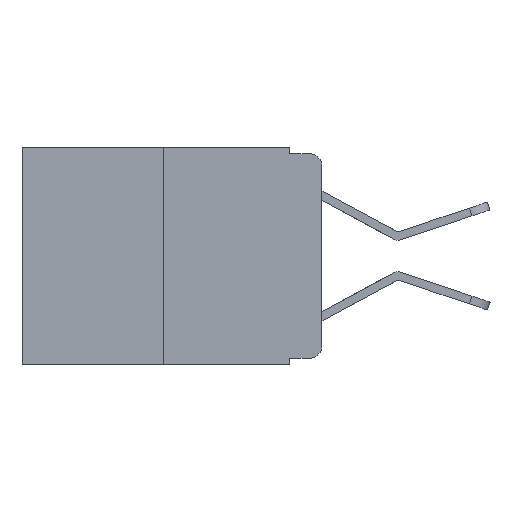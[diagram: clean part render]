
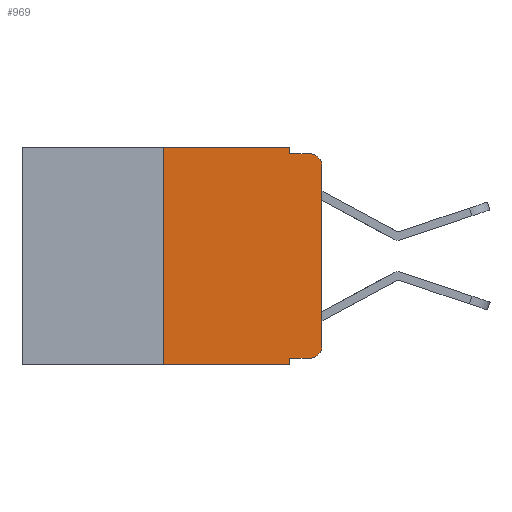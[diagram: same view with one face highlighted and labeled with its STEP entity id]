
A CAD part, left-side view. The second image highlights one B-rep face of the part: STEP entity #969.
In plain terms, the highlighted planar face has unit normal (-1, 0, 0).
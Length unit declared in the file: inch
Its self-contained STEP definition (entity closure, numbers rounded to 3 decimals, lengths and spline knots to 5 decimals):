
#143 = VECTOR ( 'NONE', #13954, 39.37008 ) ;
#254 = LINE ( 'NONE', #5528, #7622 ) ;
#380 = CARTESIAN_POINT ( 'NONE',  ( 0., 0.25, 0. ) ) ;
#518 = LINE ( 'NONE', #10164, #143 ) ;
#664 = VERTEX_POINT ( 'NONE', #6516 ) ;
#759 = AXIS2_PLACEMENT_3D ( 'NONE', #9137, #15104, #14919 ) ;
#808 = LINE ( 'NONE', #10025, #13020 ) ;
#903 = PLANE ( 'NONE',  #759 ) ;
#969 = ADVANCED_FACE ( 'NONE', ( #3757 ), #903, .F. ) ;
#1023 = CARTESIAN_POINT ( 'NONE',  ( 0., 0.051, 0. ) ) ;
#1136 = EDGE_CURVE ( 'NONE', #5374, #13135, #7244, .T. ) ;
#1180 = ORIENTED_EDGE ( 'NONE', *, *, #13018, .T. ) ;
#1422 = LINE ( 'NONE', #1023, #13125 ) ;
#3008 = CARTESIAN_POINT ( 'NONE',  ( 0., 0.02, -0.333 ) ) ;
#3103 = CIRCLE ( 'NONE', #9961, 0.02 ) ;
#3484 = CARTESIAN_POINT ( 'NONE',  ( 0., 0.051, -0.333 ) ) ;
#3704 = EDGE_CURVE ( 'NONE', #8848, #664, #3103, .T. ) ;
#3757 = FACE_OUTER_BOUND ( 'NONE', #5699, .T. ) ;
#3791 = VECTOR ( 'NONE', #14835, 39.37008 ) ;
#3911 = CARTESIAN_POINT ( 'NONE',  ( 0., 0.051, -0.01 ) ) ;
#3981 = EDGE_CURVE ( 'NONE', #11200, #5374, #14422, .T. ) ;
#4376 = DIRECTION ( 'NONE',  ( 0., 0., 1. ) ) ;
#4442 = EDGE_CURVE ( 'NONE', #4542, #13121, #1422, .T. ) ;
#4503 = LINE ( 'NONE', #380, #15077 ) ;
#4542 = VERTEX_POINT ( 'NONE', #3484 ) ;
#5076 = VECTOR ( 'NONE', #13237, 39.37008 ) ;
#5219 = VERTEX_POINT ( 'NONE', #9619 ) ;
#5374 = VERTEX_POINT ( 'NONE', #3911 ) ;
#5528 = CARTESIAN_POINT ( 'NONE',  ( 0., 0., 0. ) ) ;
#5699 = EDGE_LOOP ( 'NONE', ( #10292, #7674, #13371, #15097, #11993, #7502, #1180, #9993, #12969, #14958 ) ) ;
#6398 = CIRCLE ( 'NONE', #10613, 0.02 ) ;
#6484 = EDGE_CURVE ( 'NONE', #7038, #7924, #4503, .T. ) ;
#6516 = CARTESIAN_POINT ( 'NONE',  ( 0., 0., -0.313 ) ) ;
#6709 = LINE ( 'NONE', #12533, #3791 ) ;
#7038 = VERTEX_POINT ( 'NONE', #8792 ) ;
#7244 = LINE ( 'NONE', #12043, #5076 ) ;
#7458 = CARTESIAN_POINT ( 'NONE',  ( 0., 0.25, 0. ) ) ;
#7502 = ORIENTED_EDGE ( 'NONE', *, *, #6484, .F. ) ;
#7622 = VECTOR ( 'NONE', #4376, 39.37008 ) ;
#7674 = ORIENTED_EDGE ( 'NONE', *, *, #11751, .T. ) ;
#7924 = VERTEX_POINT ( 'NONE', #7458 ) ;
#8792 = CARTESIAN_POINT ( 'NONE',  ( 0., 0.25, -0.343 ) ) ;
#8848 = VERTEX_POINT ( 'NONE', #3008 ) ;
#8976 = DIRECTION ( 'NONE',  ( -1., 0., 0. ) ) ;
#9137 = CARTESIAN_POINT ( 'NONE',  ( 0., 0.473, 0. ) ) ;
#9619 = CARTESIAN_POINT ( 'NONE',  ( 0., 0., -0.03 ) ) ;
#9640 = DIRECTION ( 'NONE',  ( -1., 0., 0. ) ) ;
#9930 = CARTESIAN_POINT ( 'NONE',  ( 0., 0.051, 0. ) ) ;
#9961 = AXIS2_PLACEMENT_3D ( 'NONE', #10929, #9640, #10818 ) ;
#9993 = ORIENTED_EDGE ( 'NONE', *, *, #4442, .F. ) ;
#10025 = CARTESIAN_POINT ( 'NONE',  ( 0., 0.051, -0.333 ) ) ;
#10082 = EDGE_CURVE ( 'NONE', #7924, #11200, #518, .T. ) ;
#10164 = CARTESIAN_POINT ( 'NONE',  ( 0., 0.473, 0. ) ) ;
#10254 = CARTESIAN_POINT ( 'NONE',  ( 0., 0.02, -0.03 ) ) ;
#10292 = ORIENTED_EDGE ( 'NONE', *, *, #13781, .T. ) ;
#10613 = AXIS2_PLACEMENT_3D ( 'NONE', #10254, #8976, #15006 ) ;
#10818 = DIRECTION ( 'NONE',  ( 0., 0., -1. ) ) ;
#10929 = CARTESIAN_POINT ( 'NONE',  ( 0., 0.02, -0.313 ) ) ;
#11200 = VERTEX_POINT ( 'NONE', #14034 ) ;
#11751 = EDGE_CURVE ( 'NONE', #5219, #13135, #6398, .T. ) ;
#11993 = ORIENTED_EDGE ( 'NONE', *, *, #10082, .F. ) ;
#12043 = CARTESIAN_POINT ( 'NONE',  ( 0., 0.051, -0.01 ) ) ;
#12533 = CARTESIAN_POINT ( 'NONE',  ( 0., 0.473, -0.343 ) ) ;
#12588 = CARTESIAN_POINT ( 'NONE',  ( 0., 0.02, -0.01 ) ) ;
#12664 = DIRECTION ( 'NONE',  ( 0., 0., -1. ) ) ;
#12969 = ORIENTED_EDGE ( 'NONE', *, *, #13627, .T. ) ;
#13018 = EDGE_CURVE ( 'NONE', #7038, #13121, #6709, .T. ) ;
#13020 = VECTOR ( 'NONE', #13435, 39.37008 ) ;
#13121 = VERTEX_POINT ( 'NONE', #13988 ) ;
#13125 = VECTOR ( 'NONE', #12664, 39.37008 ) ;
#13135 = VERTEX_POINT ( 'NONE', #12588 ) ;
#13200 = DIRECTION ( 'NONE',  ( 0., 0., 1. ) ) ;
#13237 = DIRECTION ( 'NONE',  ( 0., -1., 0. ) ) ;
#13371 = ORIENTED_EDGE ( 'NONE', *, *, #1136, .F. ) ;
#13435 = DIRECTION ( 'NONE',  ( 0., -1., 0. ) ) ;
#13627 = EDGE_CURVE ( 'NONE', #4542, #8848, #808, .T. ) ;
#13781 = EDGE_CURVE ( 'NONE', #664, #5219, #254, .T. ) ;
#13848 = VECTOR ( 'NONE', #14646, 39.37008 ) ;
#13954 = DIRECTION ( 'NONE',  ( 0., -1., 0. ) ) ;
#13988 = CARTESIAN_POINT ( 'NONE',  ( 0., 0.051, -0.343 ) ) ;
#14034 = CARTESIAN_POINT ( 'NONE',  ( 0., 0.051, 0. ) ) ;
#14422 = LINE ( 'NONE', #9930, #13848 ) ;
#14646 = DIRECTION ( 'NONE',  ( 0., 0., -1. ) ) ;
#14835 = DIRECTION ( 'NONE',  ( 0., -1., 0. ) ) ;
#14919 = DIRECTION ( 'NONE',  ( 0., 0., -1. ) ) ;
#14958 = ORIENTED_EDGE ( 'NONE', *, *, #3704, .T. ) ;
#15006 = DIRECTION ( 'NONE',  ( 0., 0., -1. ) ) ;
#15077 = VECTOR ( 'NONE', #13200, 39.37008 ) ;
#15097 = ORIENTED_EDGE ( 'NONE', *, *, #3981, .F. ) ;
#15104 = DIRECTION ( 'NONE',  ( 1., 0., 0. ) ) ;
